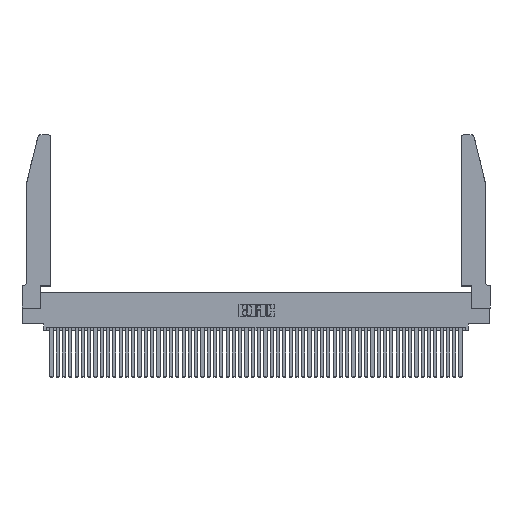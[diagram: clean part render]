
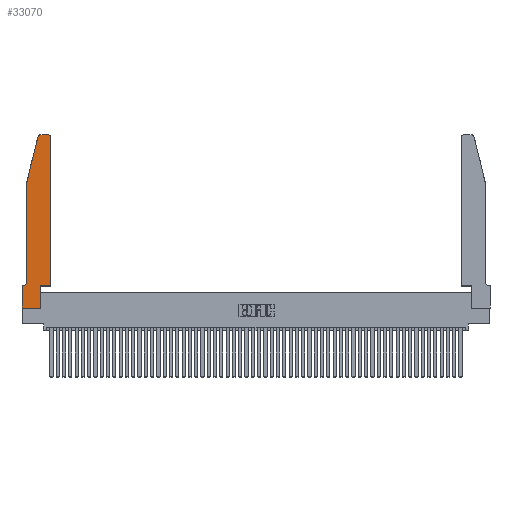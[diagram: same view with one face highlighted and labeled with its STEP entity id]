
A CAD part, top view. The second image highlights one B-rep face of the part: STEP entity #33070.
In plain terms, the highlighted planar face has unit normal (0, 0, 1).
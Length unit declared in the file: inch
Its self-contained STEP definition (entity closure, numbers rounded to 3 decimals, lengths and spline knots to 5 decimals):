
#429 = ORIENTED_EDGE ( 'NONE', *, *, #48255, .T. ) ;
#505 = EDGE_CURVE ( 'NONE', #32360, #26654, #43643, .T. ) ;
#1037 = VECTOR ( 'NONE', #39473, 39.37008 ) ;
#1128 = LINE ( 'NONE', #37324, #21955 ) ;
#1268 = AXIS2_PLACEMENT_3D ( 'NONE', #6040, #34848, #10245 ) ;
#1793 = DIRECTION ( 'NONE',  ( 0., 0., 1. ) ) ;
#2529 = LINE ( 'NONE', #21676, #45051 ) ;
#3373 = AXIS2_PLACEMENT_3D ( 'NONE', #26634, #1793, #30748 ) ;
#3797 = CARTESIAN_POINT ( 'NONE',  ( 0.4205, 2.72, 0.37 ) ) ;
#3946 = CARTESIAN_POINT ( 'NONE',  ( 0.4505, 2.72, 0.37 ) ) ;
#4224 = CARTESIAN_POINT ( 'NONE',  ( 0.2865, 0.35, 0.37 ) ) ;
#5362 = AXIS2_PLACEMENT_3D ( 'NONE', #3797, #32698, #8036 ) ;
#5656 = VECTOR ( 'NONE', #24591, 39.37008 ) ;
#5949 = DIRECTION ( 'NONE',  ( -1., 0., 0. ) ) ;
#6040 = CARTESIAN_POINT ( 'NONE',  ( 0.0055, 0.42, 0.37 ) ) ;
#6070 = DIRECTION ( 'NONE',  ( -0.239, -0.971, 0. ) ) ;
#6720 = CIRCLE ( 'NONE', #5362, 0.03 ) ;
#6737 = DIRECTION ( 'NONE',  ( 0., 0., 1. ) ) ;
#7270 = EDGE_CURVE ( 'NONE', #21073, #22657, #48212, .T. ) ;
#7568 = LINE ( 'NONE', #46883, #49878 ) ;
#8036 = DIRECTION ( 'NONE',  ( 1., 0., 0. ) ) ;
#8105 = EDGE_CURVE ( 'NONE', #26654, #47371, #23229, .T. ) ;
#9612 = CARTESIAN_POINT ( 'NONE',  ( 0., 0.35, 0.37 ) ) ;
#10245 = DIRECTION ( 'NONE',  ( -1., 0., 0. ) ) ;
#10783 = CARTESIAN_POINT ( 'NONE',  ( 0.2865, 0.35, 0.37 ) ) ;
#10941 = CARTESIAN_POINT ( 'NONE',  ( 0.4505, 0.35, 0.37 ) ) ;
#11641 = VERTEX_POINT ( 'NONE', #18609 ) ;
#12286 = VECTOR ( 'NONE', #35523, 39.37008 ) ;
#12916 = VERTEX_POINT ( 'NONE', #30870 ) ;
#13249 = EDGE_CURVE ( 'NONE', #48315, #27467, #7568, .T. ) ;
#14451 = CARTESIAN_POINT ( 'NONE',  ( 0.2865, 0., 0.37 ) ) ;
#14850 = EDGE_CURVE ( 'NONE', #35095, #12916, #6720, .T. ) ;
#17494 = ORIENTED_EDGE ( 'NONE', *, *, #44864, .T. ) ;
#17638 = VERTEX_POINT ( 'NONE', #45046 ) ;
#17756 = EDGE_CURVE ( 'NONE', #12916, #17638, #46819, .T. ) ;
#18221 = EDGE_CURVE ( 'NONE', #11641, #32360, #49331, .T. ) ;
#18609 = CARTESIAN_POINT ( 'NONE',  ( 0., 0., 0.37 ) ) ;
#20372 = LINE ( 'NONE', #41360, #36978 ) ;
#20573 = CIRCLE ( 'NONE', #3373, 0.03 ) ;
#20667 = ORIENTED_EDGE ( 'NONE', *, *, #18221, .T. ) ;
#20987 = DIRECTION ( 'NONE',  ( 0., 1., 0. ) ) ;
#21073 = VERTEX_POINT ( 'NONE', #21529 ) ;
#21529 = CARTESIAN_POINT ( 'NONE',  ( 0.25487, 2.72718, 0.37 ) ) ;
#21676 = CARTESIAN_POINT ( 'NONE',  ( 0., 0., 0.37 ) ) ;
#21955 = VECTOR ( 'NONE', #25005, 39.37008 ) ;
#22657 = VERTEX_POINT ( 'NONE', #34225 ) ;
#23188 = PLANE ( 'NONE',  #36604 ) ;
#23229 = LINE ( 'NONE', #10941, #12286 ) ;
#23829 = CARTESIAN_POINT ( 'NONE',  ( 0.4505, 0.35, 0.37 ) ) ;
#24408 = CARTESIAN_POINT ( 'NONE',  ( 0., 0., 0.37 ) ) ;
#24591 = DIRECTION ( 'NONE',  ( 1., 0., 0. ) ) ;
#25005 = DIRECTION ( 'NONE',  ( 0., -1., 0. ) ) ;
#25960 = VERTEX_POINT ( 'NONE', #36720 ) ;
#26428 = ORIENTED_EDGE ( 'NONE', *, *, #13249, .T. ) ;
#26634 = CARTESIAN_POINT ( 'NONE',  ( 0.284, 2.72, 0.37 ) ) ;
#26654 = VERTEX_POINT ( 'NONE', #4224 ) ;
#27467 = VERTEX_POINT ( 'NONE', #9612 ) ;
#30005 = EDGE_CURVE ( 'NONE', #17638, #21073, #20573, .T. ) ;
#30748 = DIRECTION ( 'NONE',  ( 1., 0., 0. ) ) ;
#30801 = CARTESIAN_POINT ( 'NONE',  ( 0.0755, 2., 0.37 ) ) ;
#30870 = CARTESIAN_POINT ( 'NONE',  ( 0.4205, 2.75, 0.37 ) ) ;
#31149 = EDGE_CURVE ( 'NONE', #27467, #11641, #2529, .T. ) ;
#31442 = CARTESIAN_POINT ( 'NONE',  ( 0., 0.35, 0.37 ) ) ;
#32360 = VERTEX_POINT ( 'NONE', #14451 ) ;
#32698 = DIRECTION ( 'NONE',  ( 0., 0., 1. ) ) ;
#33070 = ADVANCED_FACE ( 'NONE', ( #53085 ), #23188, .T. ) ;
#34225 = CARTESIAN_POINT ( 'NONE',  ( 0.0755, 2., 0.37 ) ) ;
#34848 = DIRECTION ( 'NONE',  ( 0., 0., -1. ) ) ;
#35095 = VERTEX_POINT ( 'NONE', #3946 ) ;
#35508 = DIRECTION ( 'NONE',  ( 1., 0., 0. ) ) ;
#35523 = DIRECTION ( 'NONE',  ( 1., 0., 0. ) ) ;
#35978 = VECTOR ( 'NONE', #41650, 39.37008 ) ;
#36604 = AXIS2_PLACEMENT_3D ( 'NONE', #31442, #6737, #35508 ) ;
#36720 = CARTESIAN_POINT ( 'NONE',  ( 0.0755, 0.42, 0.37 ) ) ;
#36978 = VECTOR ( 'NONE', #20987, 39.37008 ) ;
#37324 = CARTESIAN_POINT ( 'NONE',  ( 0.0755, 2., 0.37 ) ) ;
#37679 = CARTESIAN_POINT ( 'NONE',  ( 0.0055, 0.35, 0.37 ) ) ;
#39473 = DIRECTION ( 'NONE',  ( 0., 1., 0. ) ) ;
#40164 = CIRCLE ( 'NONE', #1268, 0.07 ) ;
#41144 = ORIENTED_EDGE ( 'NONE', *, *, #31149, .T. ) ;
#41360 = CARTESIAN_POINT ( 'NONE',  ( 0.4505, 0.35, 0.37 ) ) ;
#41650 = DIRECTION ( 'NONE',  ( -1., 0., 0. ) ) ;
#42207 = EDGE_LOOP ( 'NONE', ( #48730, #50005, #52564, #429, #46846, #26428, #41144, #20667, #44989, #46240, #17494, #50052 ) ) ;
#43643 = LINE ( 'NONE', #10783, #1037 ) ;
#44864 = EDGE_CURVE ( 'NONE', #47371, #35095, #20372, .T. ) ;
#44989 = ORIENTED_EDGE ( 'NONE', *, *, #505, .T. ) ;
#45046 = CARTESIAN_POINT ( 'NONE',  ( 0.284, 2.75, 0.37 ) ) ;
#45051 = VECTOR ( 'NONE', #46136, 39.37008 ) ;
#45726 = EDGE_CURVE ( 'NONE', #25960, #48315, #40164, .T. ) ;
#46136 = DIRECTION ( 'NONE',  ( 0., -1., 0. ) ) ;
#46240 = ORIENTED_EDGE ( 'NONE', *, *, #8105, .T. ) ;
#46819 = LINE ( 'NONE', #49809, #35978 ) ;
#46846 = ORIENTED_EDGE ( 'NONE', *, *, #45726, .T. ) ;
#46883 = CARTESIAN_POINT ( 'NONE',  ( 0.0755, 0.35, 0.37 ) ) ;
#47371 = VERTEX_POINT ( 'NONE', #23829 ) ;
#48212 = LINE ( 'NONE', #30801, #49495 ) ;
#48255 = EDGE_CURVE ( 'NONE', #22657, #25960, #1128, .T. ) ;
#48315 = VERTEX_POINT ( 'NONE', #37679 ) ;
#48730 = ORIENTED_EDGE ( 'NONE', *, *, #17756, .T. ) ;
#49331 = LINE ( 'NONE', #24408, #5656 ) ;
#49495 = VECTOR ( 'NONE', #6070, 39.37008 ) ;
#49809 = CARTESIAN_POINT ( 'NONE',  ( 0.2605, 2.75, 0.37 ) ) ;
#49878 = VECTOR ( 'NONE', #5949, 39.37008 ) ;
#50005 = ORIENTED_EDGE ( 'NONE', *, *, #30005, .T. ) ;
#50052 = ORIENTED_EDGE ( 'NONE', *, *, #14850, .T. ) ;
#52564 = ORIENTED_EDGE ( 'NONE', *, *, #7270, .T. ) ;
#53085 = FACE_OUTER_BOUND ( 'NONE', #42207, .T. ) ;
